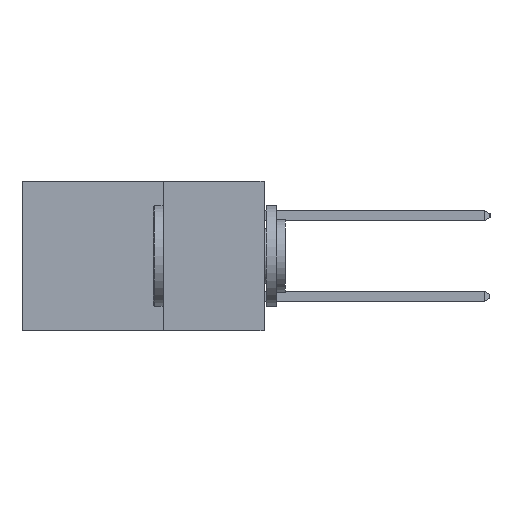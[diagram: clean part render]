
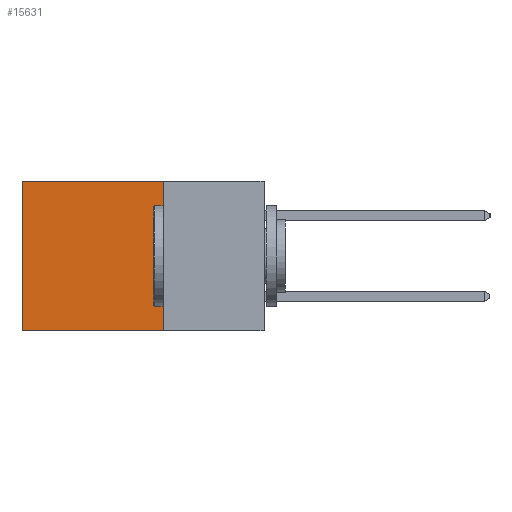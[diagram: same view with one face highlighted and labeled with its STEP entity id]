
A CAD part, left-side view. The second image highlights one B-rep face of the part: STEP entity #15631.
In plain terms, the highlighted planar face has unit normal (-1, 0, 0).
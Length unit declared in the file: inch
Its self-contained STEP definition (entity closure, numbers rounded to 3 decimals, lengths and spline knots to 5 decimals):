
#35 = CARTESIAN_POINT ( 'NONE',  ( 0.2615, 0.25, 0. ) ) ;
#176 = DIRECTION ( 'NONE',  ( 0., 0., -1. ) ) ;
#517 = DIRECTION ( 'NONE',  ( 0., 0., -1. ) ) ;
#1015 = ORIENTED_EDGE ( 'NONE', *, *, #7549, .F. ) ;
#1431 = CARTESIAN_POINT ( 'NONE',  ( 0.2615, 0.6, -0.37 ) ) ;
#1675 = LINE ( 'NONE', #6724, #10320 ) ;
#1758 = CARTESIAN_POINT ( 'NONE',  ( 0.2615, 0.25, -0.37 ) ) ;
#1760 = LINE ( 'NONE', #5728, #14930 ) ;
#1984 = EDGE_CURVE ( 'NONE', #2940, #5258, #4090, .T. ) ;
#2081 = ORIENTED_EDGE ( 'NONE', *, *, #2151, .F. ) ;
#2151 = EDGE_CURVE ( 'NONE', #2940, #5608, #1760, .T. ) ;
#2857 = DIRECTION ( 'NONE',  ( 0., 0., -1. ) ) ;
#2940 = VERTEX_POINT ( 'NONE', #3947 ) ;
#3342 = CARTESIAN_POINT ( 'NONE',  ( 0.2615, 0.6, 0. ) ) ;
#3947 = CARTESIAN_POINT ( 'NONE',  ( 0.2615, 0.25, 0. ) ) ;
#4090 = LINE ( 'NONE', #35, #14406 ) ;
#4253 = DIRECTION ( 'NONE',  ( 1., 0., 0. ) ) ;
#5258 = VERTEX_POINT ( 'NONE', #3342 ) ;
#5608 = VERTEX_POINT ( 'NONE', #15229 ) ;
#5728 = CARTESIAN_POINT ( 'NONE',  ( 0.2615, 0.25, -0.37 ) ) ;
#6316 = AXIS2_PLACEMENT_3D ( 'NONE', #1758, #4253, #2857 ) ;
#6405 = LINE ( 'NONE', #1431, #12337 ) ;
#6724 = CARTESIAN_POINT ( 'NONE',  ( 0.2615, 0.25, -0.37 ) ) ;
#7231 = ORIENTED_EDGE ( 'NONE', *, *, #1984, .T. ) ;
#7360 = CARTESIAN_POINT ( 'NONE',  ( 0.2615, 0.6, -0.37 ) ) ;
#7549 = EDGE_CURVE ( 'NONE', #5608, #10371, #1675, .T. ) ;
#8889 = EDGE_LOOP ( 'NONE', ( #11195, #1015, #2081, #7231 ) ) ;
#10320 = VECTOR ( 'NONE', #13988, 39.37008 ) ;
#10371 = VERTEX_POINT ( 'NONE', #7360 ) ;
#11195 = ORIENTED_EDGE ( 'NONE', *, *, #12040, .T. ) ;
#12040 = EDGE_CURVE ( 'NONE', #5258, #10371, #6405, .T. ) ;
#12337 = VECTOR ( 'NONE', #176, 39.37008 ) ;
#12897 = DIRECTION ( 'NONE',  ( 0., 1., 0. ) ) ;
#12982 = FACE_OUTER_BOUND ( 'NONE', #8889, .T. ) ;
#13988 = DIRECTION ( 'NONE',  ( 0., 1., 0. ) ) ;
#14228 = PLANE ( 'NONE',  #6316 ) ;
#14406 = VECTOR ( 'NONE', #12897, 39.37008 ) ;
#14930 = VECTOR ( 'NONE', #517, 39.37008 ) ;
#15229 = CARTESIAN_POINT ( 'NONE',  ( 0.2615, 0.25, -0.37 ) ) ;
#15631 = ADVANCED_FACE ( 'NONE', ( #12982 ), #14228, .F. ) ;
